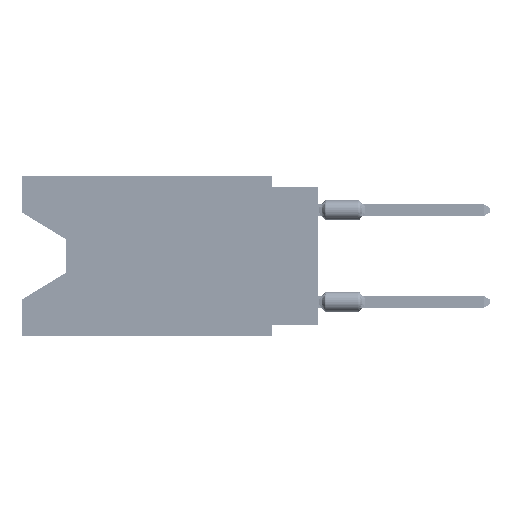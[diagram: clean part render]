
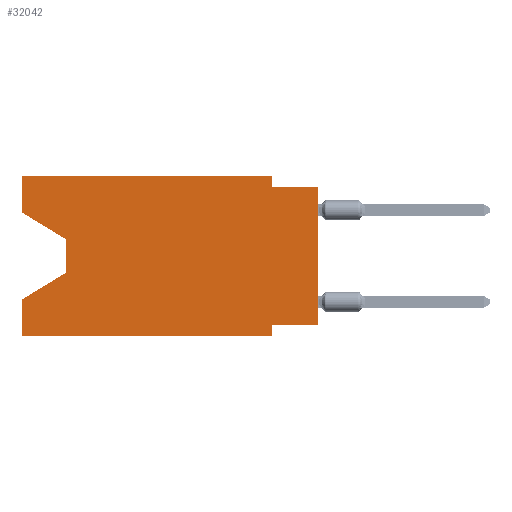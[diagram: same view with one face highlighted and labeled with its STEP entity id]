
A CAD part, left-side view. The second image highlights one B-rep face of the part: STEP entity #32042.
In plain terms, the highlighted planar face has unit normal (-1, 0, 0).
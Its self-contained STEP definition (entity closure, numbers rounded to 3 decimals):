
#1391 = EDGE_LOOP ( 'NONE', ( #30986, #60700, #53713, #48490, #24726, #5598, #2954, #23338, #3745, #79331, #47688, #26444 ) ) ;
#2479 = DIRECTION ( 'NONE',  ( 0., 0.855, -0.519 ) ) ;
#2954 = ORIENTED_EDGE ( 'NONE', *, *, #80291, .F. ) ;
#3745 = ORIENTED_EDGE ( 'NONE', *, *, #29244, .F. ) ;
#4628 = DIRECTION ( 'NONE',  ( 0., -0.855, -0.519 ) ) ;
#5598 = ORIENTED_EDGE ( 'NONE', *, *, #28656, .F. ) ;
#7484 = VECTOR ( 'NONE', #57487, 1000. ) ;
#9556 = VERTEX_POINT ( 'NONE', #42622 ) ;
#9918 = CARTESIAN_POINT ( 'NONE',  ( 0., 16.383, -2.038 ) ) ;
#10379 = CARTESIAN_POINT ( 'NONE',  ( 0., 0., -0.635 ) ) ;
#10876 = LINE ( 'NONE', #36186, #93883 ) ;
#11811 = LINE ( 'NONE', #20417, #55156 ) ;
#16327 = VECTOR ( 'NONE', #17315, 1000. ) ;
#17102 = DIRECTION ( 'NONE',  ( 0., 0., -1. ) ) ;
#17315 = DIRECTION ( 'NONE',  ( 0., 0., 1. ) ) ;
#18399 = VECTOR ( 'NONE', #28710, 1000. ) ;
#18977 = LINE ( 'NONE', #42298, #7484 ) ;
#20417 = CARTESIAN_POINT ( 'NONE',  ( 0., 16.383, 0. ) ) ;
#21204 = VERTEX_POINT ( 'NONE', #86987 ) ;
#23338 = ORIENTED_EDGE ( 'NONE', *, *, #53675, .T. ) ;
#23832 = EDGE_CURVE ( 'NONE', #84369, #27189, #94652, .T. ) ;
#24591 = CARTESIAN_POINT ( 'NONE',  ( 0., 0., -8.255 ) ) ;
#24726 = ORIENTED_EDGE ( 'NONE', *, *, #84099, .T. ) ;
#25092 = LINE ( 'NONE', #24591, #77237 ) ;
#25167 = LINE ( 'NONE', #57075, #25727 ) ;
#25727 = VECTOR ( 'NONE', #58078, 1000. ) ;
#26444 = ORIENTED_EDGE ( 'NONE', *, *, #95481, .F. ) ;
#27189 = VERTEX_POINT ( 'NONE', #64787 ) ;
#27442 = DIRECTION ( 'NONE',  ( 0., -1., 0. ) ) ;
#28542 = EDGE_CURVE ( 'NONE', #63010, #93233, #28935, .T. ) ;
#28656 = EDGE_CURVE ( 'NONE', #21204, #82571, #29940, .T. ) ;
#28710 = DIRECTION ( 'NONE',  ( 0., 0., -1. ) ) ;
#28935 = LINE ( 'NONE', #90673, #91400 ) ;
#29244 = EDGE_CURVE ( 'NONE', #90384, #73754, #87336, .T. ) ;
#29637 = CARTESIAN_POINT ( 'NONE',  ( 0., 16.383, 0. ) ) ;
#29921 = VECTOR ( 'NONE', #17102, 1000. ) ;
#29940 = LINE ( 'NONE', #38046, #29921 ) ;
#30986 = ORIENTED_EDGE ( 'NONE', *, *, #28542, .T. ) ;
#32042 = ADVANCED_FACE ( 'NONE', ( #78079 ), #32515, .F. ) ;
#32053 = CARTESIAN_POINT ( 'NONE',  ( 0., 16.383, -8.89 ) ) ;
#32515 = PLANE ( 'NONE',  #72450 ) ;
#32900 = EDGE_CURVE ( 'NONE', #9556, #90384, #25167, .T. ) ;
#35670 = EDGE_CURVE ( 'NONE', #72238, #9556, #11811, .T. ) ;
#36186 = CARTESIAN_POINT ( 'NONE',  ( 0., 16.383, 0. ) ) ;
#36810 = CARTESIAN_POINT ( 'NONE',  ( 0., 13.97, -3.505 ) ) ;
#38046 = CARTESIAN_POINT ( 'NONE',  ( 0., 2.54, -8.89 ) ) ;
#38654 = CARTESIAN_POINT ( 'NONE',  ( 0., 2.54, -8.89 ) ) ;
#42060 = CARTESIAN_POINT ( 'NONE',  ( 0., 16.383, -8.89 ) ) ;
#42298 = CARTESIAN_POINT ( 'NONE',  ( 0., 16.383, 0. ) ) ;
#42622 = CARTESIAN_POINT ( 'NONE',  ( 0., 2.54, 0. ) ) ;
#42730 = DIRECTION ( 'NONE',  ( 0., -1., 0. ) ) ;
#47688 = ORIENTED_EDGE ( 'NONE', *, *, #35670, .F. ) ;
#48490 = ORIENTED_EDGE ( 'NONE', *, *, #66815, .F. ) ;
#48892 = DIRECTION ( 'NONE',  ( 0., -1., 0. ) ) ;
#48909 = DIRECTION ( 'NONE',  ( 0., 1., 0. ) ) ;
#51391 = DIRECTION ( 'NONE',  ( 0., 0., 1. ) ) ;
#52271 = VECTOR ( 'NONE', #2479, 1000. ) ;
#53403 = VERTEX_POINT ( 'NONE', #80171 ) ;
#53675 = EDGE_CURVE ( 'NONE', #53403, #73754, #78069, .T. ) ;
#53713 = ORIENTED_EDGE ( 'NONE', *, *, #23832, .T. ) ;
#55156 = VECTOR ( 'NONE', #42730, 1000. ) ;
#55825 = DIRECTION ( 'NONE',  ( 1., 0., 0. ) ) ;
#57075 = CARTESIAN_POINT ( 'NONE',  ( 0., 2.54, 0. ) ) ;
#57330 = CARTESIAN_POINT ( 'NONE',  ( 0., 2.54, -0.635 ) ) ;
#57487 = DIRECTION ( 'NONE',  ( 0., 0., 1. ) ) ;
#58078 = DIRECTION ( 'NONE',  ( 0., 0., -1. ) ) ;
#59106 = LINE ( 'NONE', #36810, #18399 ) ;
#59576 = VECTOR ( 'NONE', #27442, 1000. ) ;
#60700 = ORIENTED_EDGE ( 'NONE', *, *, #92603, .T. ) ;
#63010 = VERTEX_POINT ( 'NONE', #9918 ) ;
#64787 = CARTESIAN_POINT ( 'NONE',  ( 0., 16.383, -6.852 ) ) ;
#64949 = CARTESIAN_POINT ( 'NONE',  ( 0., 13.97, -3.505 ) ) ;
#66815 = EDGE_CURVE ( 'NONE', #96368, #27189, #10876, .T. ) ;
#69995 = CARTESIAN_POINT ( 'NONE',  ( 0., 0., 0. ) ) ;
#72238 = VERTEX_POINT ( 'NONE', #29637 ) ;
#72450 = AXIS2_PLACEMENT_3D ( 'NONE', #94283, #55825, #86694 ) ;
#73754 = VERTEX_POINT ( 'NONE', #87287 ) ;
#77237 = VECTOR ( 'NONE', #48909, 1000. ) ;
#78069 = LINE ( 'NONE', #69995, #16327 ) ;
#78079 = FACE_OUTER_BOUND ( 'NONE', #1391, .T. ) ;
#78113 = LINE ( 'NONE', #32053, #59576 ) ;
#79331 = ORIENTED_EDGE ( 'NONE', *, *, #32900, .F. ) ;
#80171 = CARTESIAN_POINT ( 'NONE',  ( 0., 0., -8.255 ) ) ;
#80291 = EDGE_CURVE ( 'NONE', #53403, #21204, #25092, .T. ) ;
#82571 = VERTEX_POINT ( 'NONE', #38654 ) ;
#84099 = EDGE_CURVE ( 'NONE', #96368, #82571, #78113, .T. ) ;
#84369 = VERTEX_POINT ( 'NONE', #91188 ) ;
#86578 = VECTOR ( 'NONE', #48892, 1000. ) ;
#86694 = DIRECTION ( 'NONE',  ( 0., 0., -1. ) ) ;
#86987 = CARTESIAN_POINT ( 'NONE',  ( 0., 2.54, -8.255 ) ) ;
#87287 = CARTESIAN_POINT ( 'NONE',  ( 0., 0., -0.635 ) ) ;
#87336 = LINE ( 'NONE', #10379, #86578 ) ;
#90384 = VERTEX_POINT ( 'NONE', #57330 ) ;
#90673 = CARTESIAN_POINT ( 'NONE',  ( 0., 16.383, -2.038 ) ) ;
#91188 = CARTESIAN_POINT ( 'NONE',  ( 0., 13.97, -5.385 ) ) ;
#91400 = VECTOR ( 'NONE', #4628, 1000. ) ;
#92603 = EDGE_CURVE ( 'NONE', #93233, #84369, #59106, .T. ) ;
#93233 = VERTEX_POINT ( 'NONE', #64949 ) ;
#93883 = VECTOR ( 'NONE', #51391, 1000. ) ;
#94283 = CARTESIAN_POINT ( 'NONE',  ( 0., 16.383, 0. ) ) ;
#94652 = LINE ( 'NONE', #95151, #52271 ) ;
#95151 = CARTESIAN_POINT ( 'NONE',  ( 0., 13.97, -5.385 ) ) ;
#95481 = EDGE_CURVE ( 'NONE', #63010, #72238, #18977, .T. ) ;
#96368 = VERTEX_POINT ( 'NONE', #42060 ) ;
